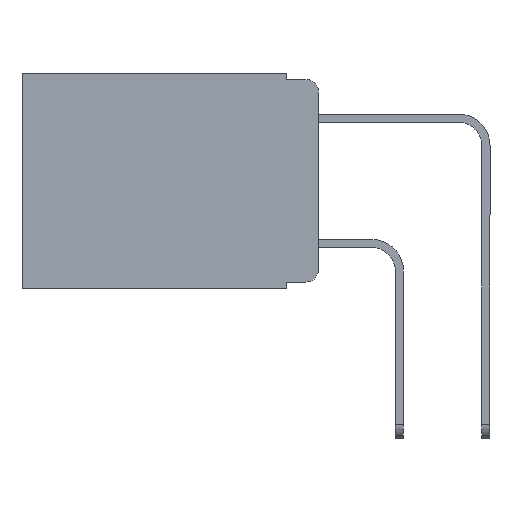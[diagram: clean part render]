
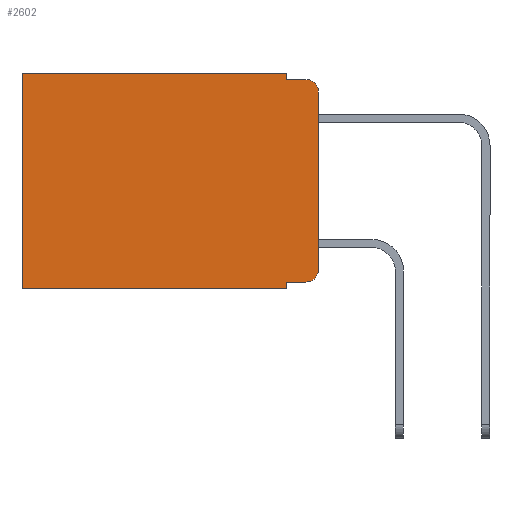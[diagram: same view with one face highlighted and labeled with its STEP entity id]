
A CAD part, left-side view. The second image highlights one B-rep face of the part: STEP entity #2602.
In plain terms, the highlighted planar face has unit normal (-1, 0, 0).
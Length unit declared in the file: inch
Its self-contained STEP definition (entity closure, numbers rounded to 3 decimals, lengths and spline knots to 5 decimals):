
#52 = VERTEX_POINT ( 'NONE', #8028 ) ;
#286 = VECTOR ( 'NONE', #4516, 39.37008 ) ;
#402 = EDGE_CURVE ( 'NONE', #6683, #5652, #8088, .T. ) ;
#470 = CARTESIAN_POINT ( 'NONE',  ( 0.298, 0.02, -0.333 ) ) ;
#1313 = CARTESIAN_POINT ( 'NONE',  ( 0.298, 0.473, -0.343 ) ) ;
#1382 = CIRCLE ( 'NONE', #10632, 0.02 ) ;
#1485 = CARTESIAN_POINT ( 'NONE',  ( 0.298, 0., 0. ) ) ;
#1632 = VERTEX_POINT ( 'NONE', #2865 ) ;
#1835 = CARTESIAN_POINT ( 'NONE',  ( 0.298, 0.051, -0.333 ) ) ;
#1861 = EDGE_CURVE ( 'NONE', #3045, #5507, #7628, .T. ) ;
#1988 = EDGE_CURVE ( 'NONE', #1632, #3045, #8363, .T. ) ;
#2019 = LINE ( 'NONE', #4821, #7010 ) ;
#2101 = CARTESIAN_POINT ( 'NONE',  ( 0.298, 0., -0.343 ) ) ;
#2356 = EDGE_CURVE ( 'NONE', #4524, #52, #10495, .T. ) ;
#2596 = DIRECTION ( 'NONE',  ( 0., 1., 0. ) ) ;
#2602 = ADVANCED_FACE ( 'NONE', ( #2978 ), #4014, .F. ) ;
#2791 = DIRECTION ( 'NONE',  ( -1., 0., 0. ) ) ;
#2810 = DIRECTION ( 'NONE',  ( 0., 0., -1. ) ) ;
#2828 = VECTOR ( 'NONE', #9665, 39.37008 ) ;
#2837 = LINE ( 'NONE', #11016, #10503 ) ;
#2865 = CARTESIAN_POINT ( 'NONE',  ( 0.298, 0.051, 0. ) ) ;
#2978 = FACE_OUTER_BOUND ( 'NONE', #4992, .T. ) ;
#3045 = VERTEX_POINT ( 'NONE', #4586 ) ;
#3167 = VECTOR ( 'NONE', #2596, 39.37008 ) ;
#3279 = VECTOR ( 'NONE', #8332, 39.37008 ) ;
#3425 = DIRECTION ( 'NONE',  ( -1., 0., 0. ) ) ;
#3562 = EDGE_CURVE ( 'NONE', #7790, #5507, #5345, .T. ) ;
#3761 = ORIENTED_EDGE ( 'NONE', *, *, #7798, .T. ) ;
#3865 = ORIENTED_EDGE ( 'NONE', *, *, #2356, .F. ) ;
#3972 = ORIENTED_EDGE ( 'NONE', *, *, #402, .F. ) ;
#4014 = PLANE ( 'NONE',  #9590 ) ;
#4147 = VECTOR ( 'NONE', #10500, 39.37008 ) ;
#4157 = DIRECTION ( 'NONE',  ( 0., 0., -1. ) ) ;
#4229 = VERTEX_POINT ( 'NONE', #470 ) ;
#4413 = DIRECTION ( 'NONE',  ( 0., 0., -1. ) ) ;
#4516 = DIRECTION ( 'NONE',  ( 0., 0., -1. ) ) ;
#4524 = VERTEX_POINT ( 'NONE', #10976 ) ;
#4586 = CARTESIAN_POINT ( 'NONE',  ( 0.298, 0.473, 0. ) ) ;
#4692 = DIRECTION ( 'NONE',  ( 1., 0., 0. ) ) ;
#4821 = CARTESIAN_POINT ( 'NONE',  ( 0.298, 0.051, 0. ) ) ;
#4852 = CARTESIAN_POINT ( 'NONE',  ( 0.298, 0., -0.313 ) ) ;
#4992 = EDGE_LOOP ( 'NONE', ( #3972, #3761, #3865, #6237, #6176, #6309, #6242, #6391, #6376, #6521 ) ) ;
#5297 = DIRECTION ( 'NONE',  ( 0., 0., -1. ) ) ;
#5345 = LINE ( 'NONE', #2101, #3279 ) ;
#5381 = CARTESIAN_POINT ( 'NONE',  ( 0.298, 0.051, -0.343 ) ) ;
#5507 = VERTEX_POINT ( 'NONE', #1313 ) ;
#5652 = VERTEX_POINT ( 'NONE', #4852 ) ;
#6163 = EDGE_CURVE ( 'NONE', #4229, #5652, #11246, .T. ) ;
#6176 = ORIENTED_EDGE ( 'NONE', *, *, #1988, .T. ) ;
#6237 = ORIENTED_EDGE ( 'NONE', *, *, #10488, .F. ) ;
#6242 = ORIENTED_EDGE ( 'NONE', *, *, #3562, .F. ) ;
#6309 = ORIENTED_EDGE ( 'NONE', *, *, #1861, .T. ) ;
#6376 = ORIENTED_EDGE ( 'NONE', *, *, #11511, .T. ) ;
#6391 = ORIENTED_EDGE ( 'NONE', *, *, #8963, .F. ) ;
#6521 = ORIENTED_EDGE ( 'NONE', *, *, #6163, .T. ) ;
#6534 = CARTESIAN_POINT ( 'NONE',  ( 0.298, 0., 0. ) ) ;
#6683 = VERTEX_POINT ( 'NONE', #10314 ) ;
#7010 = VECTOR ( 'NONE', #2810, 39.37008 ) ;
#7628 = LINE ( 'NONE', #10482, #9794 ) ;
#7790 = VERTEX_POINT ( 'NONE', #5381 ) ;
#7798 = EDGE_CURVE ( 'NONE', #6683, #52, #1382, .T. ) ;
#8028 = CARTESIAN_POINT ( 'NONE',  ( 0.298, 0.02, -0.01 ) ) ;
#8088 = LINE ( 'NONE', #6534, #286 ) ;
#8319 = AXIS2_PLACEMENT_3D ( 'NONE', #8656, #2791, #9561 ) ;
#8332 = DIRECTION ( 'NONE',  ( 0., 1., 0. ) ) ;
#8363 = LINE ( 'NONE', #1485, #3167 ) ;
#8656 = CARTESIAN_POINT ( 'NONE',  ( 0.298, 0.02, -0.313 ) ) ;
#8963 = EDGE_CURVE ( 'NONE', #9101, #7790, #2837, .T. ) ;
#9101 = VERTEX_POINT ( 'NONE', #11992 ) ;
#9208 = CARTESIAN_POINT ( 'NONE',  ( 0.298, 0.02, -0.03 ) ) ;
#9561 = DIRECTION ( 'NONE',  ( 0., 0., -1. ) ) ;
#9590 = AXIS2_PLACEMENT_3D ( 'NONE', #11139, #4692, #5297 ) ;
#9665 = DIRECTION ( 'NONE',  ( 0., -1., 0. ) ) ;
#9794 = VECTOR ( 'NONE', #4157, 39.37008 ) ;
#10137 = DIRECTION ( 'NONE',  ( 0., 0., -1. ) ) ;
#10314 = CARTESIAN_POINT ( 'NONE',  ( 0.298, 0., -0.03 ) ) ;
#10482 = CARTESIAN_POINT ( 'NONE',  ( 0.298, 0.473, 0. ) ) ;
#10488 = EDGE_CURVE ( 'NONE', #1632, #4524, #2019, .T. ) ;
#10495 = LINE ( 'NONE', #11227, #2828 ) ;
#10500 = DIRECTION ( 'NONE',  ( 0., -1., 0. ) ) ;
#10503 = VECTOR ( 'NONE', #4413, 39.37008 ) ;
#10632 = AXIS2_PLACEMENT_3D ( 'NONE', #9208, #3425, #10137 ) ;
#10976 = CARTESIAN_POINT ( 'NONE',  ( 0.298, 0.051, -0.01 ) ) ;
#11016 = CARTESIAN_POINT ( 'NONE',  ( 0.298, 0.051, 0. ) ) ;
#11139 = CARTESIAN_POINT ( 'NONE',  ( 0.298, 0., 0. ) ) ;
#11227 = CARTESIAN_POINT ( 'NONE',  ( 0.298, 0.051, -0.01 ) ) ;
#11246 = CIRCLE ( 'NONE', #8319, 0.02 ) ;
#11511 = EDGE_CURVE ( 'NONE', #9101, #4229, #11622, .T. ) ;
#11622 = LINE ( 'NONE', #1835, #4147 ) ;
#11992 = CARTESIAN_POINT ( 'NONE',  ( 0.298, 0.051, -0.333 ) ) ;
